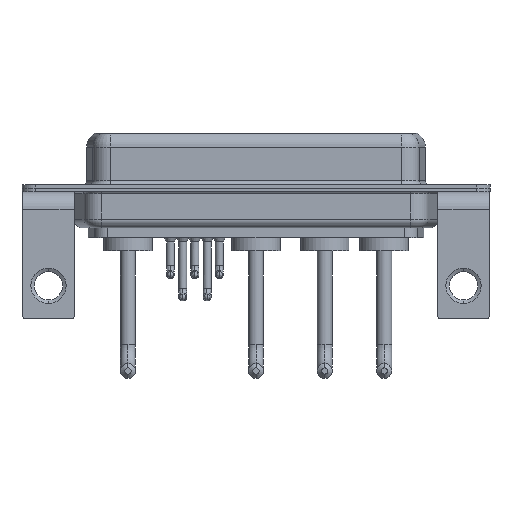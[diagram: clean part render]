
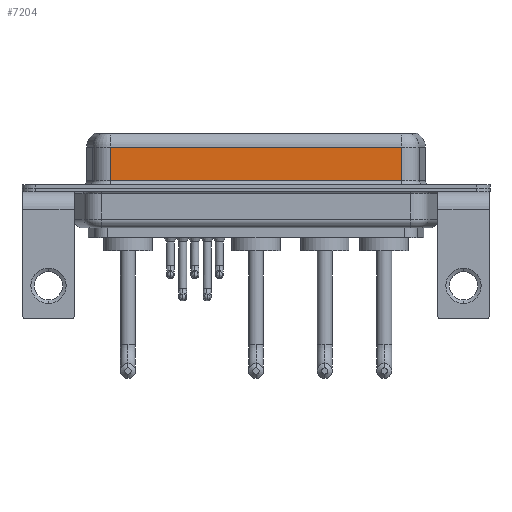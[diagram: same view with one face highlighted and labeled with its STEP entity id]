
A CAD part, front view. The second image highlights one B-rep face of the part: STEP entity #7204.
In plain terms, the highlighted planar face has unit normal (0, -1, 0).
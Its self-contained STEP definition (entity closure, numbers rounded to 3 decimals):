
#973 = VECTOR ( 'NONE', #10783, 1000. ) ;
#1029 = EDGE_CURVE ( 'NONE', #5103, #3947, #3030, .T. ) ;
#1039 = ORIENTED_EDGE ( 'NONE', *, *, #17247, .T. ) ;
#1119 = DIRECTION ( 'NONE',  ( 0., 0., -1. ) ) ;
#1129 = ORIENTED_EDGE ( 'NONE', *, *, #9763, .T. ) ;
#1255 = CARTESIAN_POINT ( 'NONE',  ( 7.013, -3.95, 0.9 ) ) ;
#1569 = FACE_OUTER_BOUND ( 'NONE', #11800, .T. ) ;
#1655 = CARTESIAN_POINT ( 'NONE',  ( 7.013, -3.95, 4.65 ) ) ;
#2552 = VECTOR ( 'NONE', #1119, 1000. ) ;
#2842 = ORIENTED_EDGE ( 'NONE', *, *, #1029, .F. ) ;
#3030 = LINE ( 'NONE', #7487, #5252 ) ;
#3387 = AXIS2_PLACEMENT_3D ( 'NONE', #13982, #11320, #5861 ) ;
#3947 = VERTEX_POINT ( 'NONE', #13539 ) ;
#5103 = VERTEX_POINT ( 'NONE', #6181 ) ;
#5225 = CARTESIAN_POINT ( 'NONE',  ( 40.037, -3.95, 0.9 ) ) ;
#5252 = VECTOR ( 'NONE', #17157, 1000. ) ;
#5493 = LINE ( 'NONE', #16615, #2552 ) ;
#5861 = DIRECTION ( 'NONE',  ( 0., 0., 1. ) ) ;
#5879 = VERTEX_POINT ( 'NONE', #1655 ) ;
#6181 = CARTESIAN_POINT ( 'NONE',  ( 40.037, -3.95, 4.65 ) ) ;
#7137 = PLANE ( 'NONE',  #3387 ) ;
#7204 = ADVANCED_FACE ( 'NONE', ( #1569 ), #7137, .F. ) ;
#7487 = CARTESIAN_POINT ( 'NONE',  ( 40.037, -3.95, 6.4 ) ) ;
#7691 = CARTESIAN_POINT ( 'NONE',  ( 40.037, -3.95, 4.65 ) ) ;
#9674 = VECTOR ( 'NONE', #14552, 1000. ) ;
#9763 = EDGE_CURVE ( 'NONE', #5879, #10075, #5493, .T. ) ;
#10075 = VERTEX_POINT ( 'NONE', #1255 ) ;
#10783 = DIRECTION ( 'NONE',  ( 1., 0., 0. ) ) ;
#11320 = DIRECTION ( 'NONE',  ( 0., 1., 0. ) ) ;
#11800 = EDGE_LOOP ( 'NONE', ( #2842, #1039, #1129, #12986 ) ) ;
#12155 = LINE ( 'NONE', #5225, #973 ) ;
#12986 = ORIENTED_EDGE ( 'NONE', *, *, #17519, .T. ) ;
#13539 = CARTESIAN_POINT ( 'NONE',  ( 40.037, -3.95, 0.9 ) ) ;
#13982 = CARTESIAN_POINT ( 'NONE',  ( 40.037, -3.95, 6.4 ) ) ;
#14552 = DIRECTION ( 'NONE',  ( -1., 0., 0. ) ) ;
#15731 = LINE ( 'NONE', #7691, #9674 ) ;
#16615 = CARTESIAN_POINT ( 'NONE',  ( 7.013, -3.95, 6.4 ) ) ;
#17157 = DIRECTION ( 'NONE',  ( 0., 0., -1. ) ) ;
#17247 = EDGE_CURVE ( 'NONE', #5103, #5879, #15731, .T. ) ;
#17519 = EDGE_CURVE ( 'NONE', #10075, #3947, #12155, .T. ) ;
